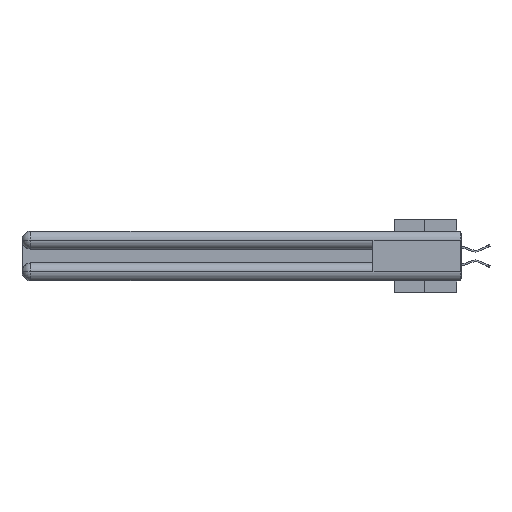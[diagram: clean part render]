
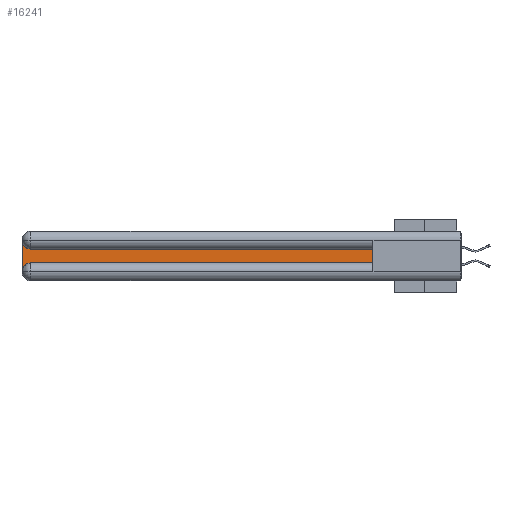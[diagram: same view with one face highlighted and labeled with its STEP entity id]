
A CAD part, left-side view. The second image highlights one B-rep face of the part: STEP entity #16241.
In plain terms, the highlighted planar face has unit normal (-1, 0, 0).
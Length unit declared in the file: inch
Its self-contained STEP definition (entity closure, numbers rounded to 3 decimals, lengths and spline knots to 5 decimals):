
#400 = DIRECTION ( 'NONE',  ( 1., 0., 0. ) ) ;
#972 = ORIENTED_EDGE ( 'NONE', *, *, #22420, .T. ) ;
#1348 = LINE ( 'NONE', #26052, #13680 ) ;
#1973 = VERTEX_POINT ( 'NONE', #42982 ) ;
#3519 = EDGE_CURVE ( 'NONE', #16582, #5214, #1348, .T. ) ;
#4226 = LINE ( 'NONE', #25549, #9559 ) ;
#4491 = VERTEX_POINT ( 'NONE', #22121 ) ;
#4681 = AXIS2_PLACEMENT_3D ( 'NONE', #16506, #27181, #30330 ) ;
#5214 = VERTEX_POINT ( 'NONE', #12831 ) ;
#7436 = LINE ( 'NONE', #36424, #13291 ) ;
#7587 = VECTOR ( 'NONE', #43094, 39.37008 ) ;
#7925 = EDGE_LOOP ( 'NONE', ( #972, #34584, #10624, #25292, #32472, #8008 ) ) ;
#8008 = ORIENTED_EDGE ( 'NONE', *, *, #3519, .T. ) ;
#9559 = VECTOR ( 'NONE', #21511, 39.37008 ) ;
#10624 = ORIENTED_EDGE ( 'NONE', *, *, #20943, .T. ) ;
#12659 = AXIS2_PLACEMENT_3D ( 'NONE', #24776, #400, #17876 ) ;
#12831 = CARTESIAN_POINT ( 'NONE',  ( 0.075, 0.6, -0.1225 ) ) ;
#13291 = VECTOR ( 'NONE', #22205, 39.37008 ) ;
#13475 = CIRCLE ( 'NONE', #21140, 0.06 ) ;
#13680 = VECTOR ( 'NONE', #22163, 39.37008 ) ;
#14170 = FACE_OUTER_BOUND ( 'NONE', #7925, .T. ) ;
#15001 = CARTESIAN_POINT ( 'NONE',  ( 0.075, 2.94, -0.2175 ) ) ;
#15663 = DIRECTION ( 'NONE',  ( 0., 0., -1. ) ) ;
#16241 = ADVANCED_FACE ( 'NONE', ( #14170 ), #41699, .F. ) ;
#16506 = CARTESIAN_POINT ( 'NONE',  ( 0.075, 2.94, -0.0625 ) ) ;
#16582 = VERTEX_POINT ( 'NONE', #35355 ) ;
#17876 = DIRECTION ( 'NONE',  ( 0., 0., -1. ) ) ;
#17979 = EDGE_CURVE ( 'NONE', #4491, #19861, #24879, .T. ) ;
#18054 = CARTESIAN_POINT ( 'NONE',  ( 0.075, 3., -0.0625 ) ) ;
#18267 = EDGE_CURVE ( 'NONE', #1973, #42384, #13475, .T. ) ;
#19861 = VERTEX_POINT ( 'NONE', #18054 ) ;
#20943 = EDGE_CURVE ( 'NONE', #19861, #1973, #44045, .T. ) ;
#21140 = AXIS2_PLACEMENT_3D ( 'NONE', #23034, #36397, #15663 ) ;
#21511 = DIRECTION ( 'NONE',  ( 0., 1., 0. ) ) ;
#22121 = CARTESIAN_POINT ( 'NONE',  ( 0.075, 2.94, -0.1225 ) ) ;
#22163 = DIRECTION ( 'NONE',  ( 0., 0., 1. ) ) ;
#22205 = DIRECTION ( 'NONE',  ( 0., -1., 0. ) ) ;
#22420 = EDGE_CURVE ( 'NONE', #5214, #4491, #4226, .T. ) ;
#23034 = CARTESIAN_POINT ( 'NONE',  ( 0.075, 2.94, -0.2775 ) ) ;
#24776 = CARTESIAN_POINT ( 'NONE',  ( 0.075, 3., -0.1225 ) ) ;
#24879 = CIRCLE ( 'NONE', #4681, 0.06 ) ;
#25292 = ORIENTED_EDGE ( 'NONE', *, *, #18267, .T. ) ;
#25549 = CARTESIAN_POINT ( 'NONE',  ( 0.075, 0.6, -0.1225 ) ) ;
#26052 = CARTESIAN_POINT ( 'NONE',  ( 0.075, 0.6, -0.2175 ) ) ;
#27181 = DIRECTION ( 'NONE',  ( 1., 0., 0. ) ) ;
#30330 = DIRECTION ( 'NONE',  ( 0., 0., -1. ) ) ;
#32349 = CARTESIAN_POINT ( 'NONE',  ( 0.075, 3., -0.2175 ) ) ;
#32472 = ORIENTED_EDGE ( 'NONE', *, *, #35427, .T. ) ;
#34584 = ORIENTED_EDGE ( 'NONE', *, *, #17979, .T. ) ;
#35355 = CARTESIAN_POINT ( 'NONE',  ( 0.075, 0.6, -0.2175 ) ) ;
#35427 = EDGE_CURVE ( 'NONE', #42384, #16582, #7436, .T. ) ;
#36397 = DIRECTION ( 'NONE',  ( 1., 0., 0. ) ) ;
#36424 = CARTESIAN_POINT ( 'NONE',  ( 0.075, 0.6, -0.2175 ) ) ;
#41699 = PLANE ( 'NONE',  #12659 ) ;
#42384 = VERTEX_POINT ( 'NONE', #15001 ) ;
#42982 = CARTESIAN_POINT ( 'NONE',  ( 0.075, 3., -0.2775 ) ) ;
#43094 = DIRECTION ( 'NONE',  ( 0., 0., -1. ) ) ;
#44045 = LINE ( 'NONE', #32349, #7587 ) ;
